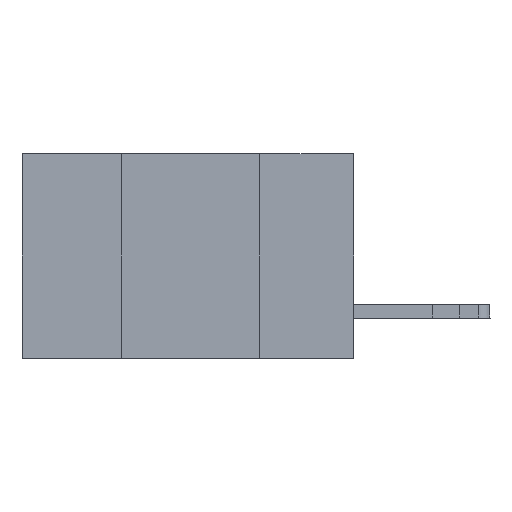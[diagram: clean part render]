
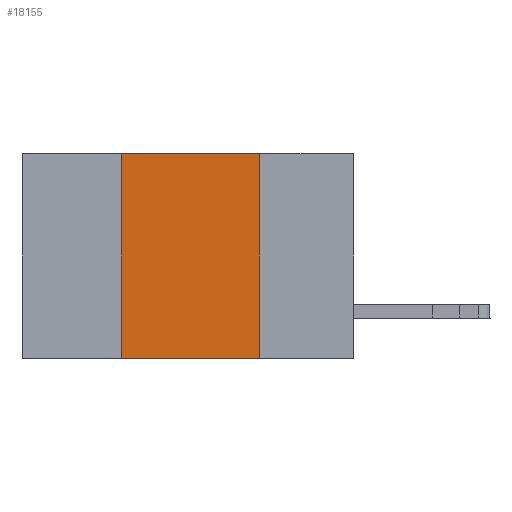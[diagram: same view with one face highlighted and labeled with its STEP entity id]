
A CAD part, left-side view. The second image highlights one B-rep face of the part: STEP entity #18155.
In plain terms, the highlighted planar face has unit normal (-1, 0, 0).
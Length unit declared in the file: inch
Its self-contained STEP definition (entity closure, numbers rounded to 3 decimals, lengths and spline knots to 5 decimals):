
#511 = DIRECTION ( 'NONE',  ( 0., 0., -1. ) ) ;
#1851 = LINE ( 'NONE', #15042, #8040 ) ;
#1922 = EDGE_CURVE ( 'NONE', #30573, #19945, #3920, .T. ) ;
#2919 = LINE ( 'NONE', #14029, #28838 ) ;
#3455 = CARTESIAN_POINT ( 'NONE',  ( 0., 0.17, 0. ) ) ;
#3920 = LINE ( 'NONE', #5414, #30624 ) ;
#5414 = CARTESIAN_POINT ( 'NONE',  ( 0., 0.6, -0.37 ) ) ;
#5857 = AXIS2_PLACEMENT_3D ( 'NONE', #13484, #16075, #511 ) ;
#6223 = DIRECTION ( 'NONE',  ( 0., 0., -1. ) ) ;
#7655 = CARTESIAN_POINT ( 'NONE',  ( 0., 0.42, 0. ) ) ;
#8040 = VECTOR ( 'NONE', #25298, 39.37008 ) ;
#8962 = ORIENTED_EDGE ( 'NONE', *, *, #1922, .T. ) ;
#10171 = CARTESIAN_POINT ( 'NONE',  ( 0., 0.42, -0.37 ) ) ;
#10696 = EDGE_CURVE ( 'NONE', #30573, #21708, #11563, .T. ) ;
#10915 = PLANE ( 'NONE',  #5857 ) ;
#10927 = VERTEX_POINT ( 'NONE', #3455 ) ;
#11009 = FACE_OUTER_BOUND ( 'NONE', #32192, .T. ) ;
#11563 = LINE ( 'NONE', #7655, #18379 ) ;
#13234 = DIRECTION ( 'NONE',  ( 0., -1., 0. ) ) ;
#13484 = CARTESIAN_POINT ( 'NONE',  ( 0., 0.6, 0. ) ) ;
#14029 = CARTESIAN_POINT ( 'NONE',  ( 0., 0.17, 0. ) ) ;
#14425 = EDGE_CURVE ( 'NONE', #21708, #10927, #1851, .T. ) ;
#15042 = CARTESIAN_POINT ( 'NONE',  ( 0., 0.6, 0. ) ) ;
#15719 = ORIENTED_EDGE ( 'NONE', *, *, #14425, .F. ) ;
#16075 = DIRECTION ( 'NONE',  ( 1., 0., 0. ) ) ;
#17885 = DIRECTION ( 'NONE',  ( 0., 0., 1. ) ) ;
#18155 = ADVANCED_FACE ( 'NONE', ( #11009 ), #10915, .F. ) ;
#18379 = VECTOR ( 'NONE', #17885, 39.37008 ) ;
#19945 = VERTEX_POINT ( 'NONE', #26922 ) ;
#21708 = VERTEX_POINT ( 'NONE', #29097 ) ;
#22932 = ORIENTED_EDGE ( 'NONE', *, *, #29682, .F. ) ;
#25298 = DIRECTION ( 'NONE',  ( 0., -1., 0. ) ) ;
#26922 = CARTESIAN_POINT ( 'NONE',  ( 0., 0.17, -0.37 ) ) ;
#28838 = VECTOR ( 'NONE', #6223, 39.37008 ) ;
#29097 = CARTESIAN_POINT ( 'NONE',  ( 0., 0.42, 0. ) ) ;
#29682 = EDGE_CURVE ( 'NONE', #10927, #19945, #2919, .T. ) ;
#29873 = ORIENTED_EDGE ( 'NONE', *, *, #10696, .F. ) ;
#30573 = VERTEX_POINT ( 'NONE', #10171 ) ;
#30624 = VECTOR ( 'NONE', #13234, 39.37008 ) ;
#32192 = EDGE_LOOP ( 'NONE', ( #22932, #15719, #29873, #8962 ) ) ;
